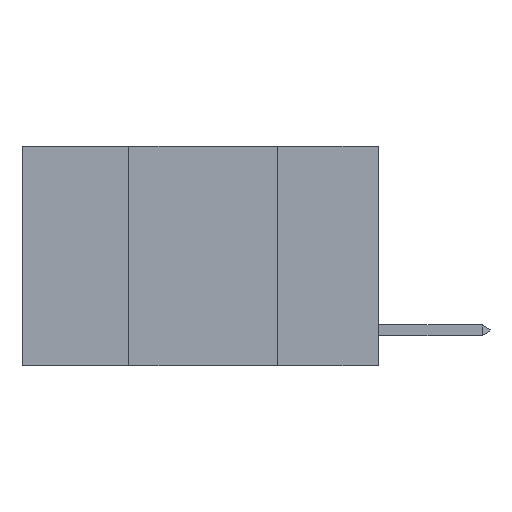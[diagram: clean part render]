
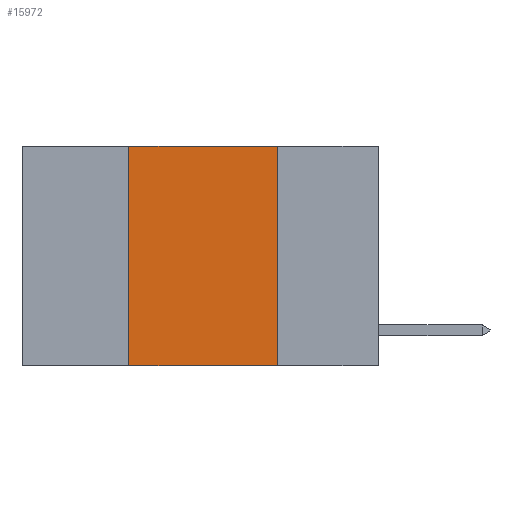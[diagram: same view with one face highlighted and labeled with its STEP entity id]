
A CAD part, left-side view. The second image highlights one B-rep face of the part: STEP entity #15972.
In plain terms, the highlighted planar face has unit normal (-1, 0, 0).
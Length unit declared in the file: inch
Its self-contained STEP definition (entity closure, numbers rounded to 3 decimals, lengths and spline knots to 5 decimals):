
#753 = DIRECTION ( 'NONE',  ( 0., -1., 0. ) ) ;
#988 = CARTESIAN_POINT ( 'NONE',  ( 0., 0.6, -0.37 ) ) ;
#1130 = EDGE_CURVE ( 'NONE', #10914, #26328, #19759, .T. ) ;
#1878 = VERTEX_POINT ( 'NONE', #24740 ) ;
#2647 = ORIENTED_EDGE ( 'NONE', *, *, #26348, .T. ) ;
#3529 = PLANE ( 'NONE',  #3872 ) ;
#3612 = DIRECTION ( 'NONE',  ( 0., 0., -1. ) ) ;
#3872 = AXIS2_PLACEMENT_3D ( 'NONE', #25327, #4546, #17485 ) ;
#3873 = CARTESIAN_POINT ( 'NONE',  ( 0., 0.42, -0.37 ) ) ;
#4546 = DIRECTION ( 'NONE',  ( 1., 0., 0. ) ) ;
#4831 = VECTOR ( 'NONE', #20509, 39.37008 ) ;
#5501 = EDGE_LOOP ( 'NONE', ( #18219, #6695, #9396, #2647 ) ) ;
#6695 = ORIENTED_EDGE ( 'NONE', *, *, #17975, .F. ) ;
#7818 = LINE ( 'NONE', #988, #24664 ) ;
#7884 = LINE ( 'NONE', #26533, #28583 ) ;
#9100 = FACE_OUTER_BOUND ( 'NONE', #5501, .T. ) ;
#9396 = ORIENTED_EDGE ( 'NONE', *, *, #1130, .F. ) ;
#9699 = CARTESIAN_POINT ( 'NONE',  ( 0., 0.17, 0. ) ) ;
#10264 = VECTOR ( 'NONE', #753, 39.37008 ) ;
#10914 = VERTEX_POINT ( 'NONE', #3873 ) ;
#14330 = DIRECTION ( 'NONE',  ( 0., -1., 0. ) ) ;
#15972 = ADVANCED_FACE ( 'NONE', ( #9100 ), #3529, .F. ) ;
#16537 = CARTESIAN_POINT ( 'NONE',  ( 0., 0.6, 0. ) ) ;
#17485 = DIRECTION ( 'NONE',  ( 0., 0., -1. ) ) ;
#17975 = EDGE_CURVE ( 'NONE', #26328, #26496, #21519, .T. ) ;
#18219 = ORIENTED_EDGE ( 'NONE', *, *, #29154, .F. ) ;
#19759 = LINE ( 'NONE', #20206, #4831 ) ;
#20206 = CARTESIAN_POINT ( 'NONE',  ( 0., 0.42, 0. ) ) ;
#20509 = DIRECTION ( 'NONE',  ( 0., 0., 1. ) ) ;
#21519 = LINE ( 'NONE', #16537, #10264 ) ;
#24664 = VECTOR ( 'NONE', #14330, 39.37008 ) ;
#24740 = CARTESIAN_POINT ( 'NONE',  ( 0., 0.17, -0.37 ) ) ;
#25327 = CARTESIAN_POINT ( 'NONE',  ( 0., 0.6, 0. ) ) ;
#26328 = VERTEX_POINT ( 'NONE', #26514 ) ;
#26348 = EDGE_CURVE ( 'NONE', #10914, #1878, #7818, .T. ) ;
#26496 = VERTEX_POINT ( 'NONE', #9699 ) ;
#26514 = CARTESIAN_POINT ( 'NONE',  ( 0., 0.42, 0. ) ) ;
#26533 = CARTESIAN_POINT ( 'NONE',  ( 0., 0.17, 0. ) ) ;
#28583 = VECTOR ( 'NONE', #3612, 39.37008 ) ;
#29154 = EDGE_CURVE ( 'NONE', #26496, #1878, #7884, .T. ) ;
